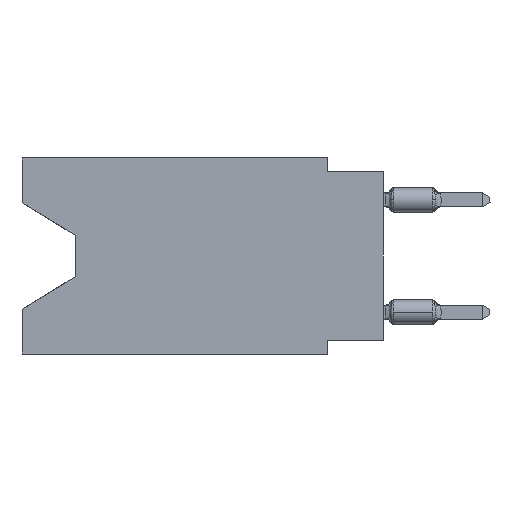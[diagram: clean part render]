
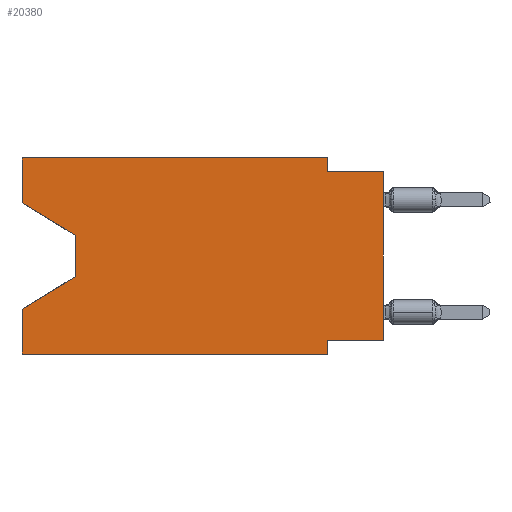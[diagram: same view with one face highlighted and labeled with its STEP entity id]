
A CAD part, left-side view. The second image highlights one B-rep face of the part: STEP entity #20380.
In plain terms, the highlighted planar face has unit normal (-1, 0, 0).
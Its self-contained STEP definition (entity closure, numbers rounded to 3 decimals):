
#86 = CARTESIAN_POINT ( 'NONE',  ( 0., 13.97, -3.505 ) ) ;
#268 = EDGE_CURVE ( 'NONE', #17791, #15368, #21144, .T. ) ;
#581 = CARTESIAN_POINT ( 'NONE',  ( 0., 2.54, 0. ) ) ;
#879 = LINE ( 'NONE', #1012, #8076 ) ;
#906 = CARTESIAN_POINT ( 'NONE',  ( 0., 16.383, -8.89 ) ) ;
#975 = VECTOR ( 'NONE', #2533, 1000. ) ;
#1012 = CARTESIAN_POINT ( 'NONE',  ( 0., 13.97, -3.505 ) ) ;
#1935 = CARTESIAN_POINT ( 'NONE',  ( 0., 16.383, -2.038 ) ) ;
#2030 = ORIENTED_EDGE ( 'NONE', *, *, #5753, .T. ) ;
#2533 = DIRECTION ( 'NONE',  ( 0., 0., 1. ) ) ;
#2632 = CARTESIAN_POINT ( 'NONE',  ( 0., 13.97, -5.385 ) ) ;
#2776 = EDGE_CURVE ( 'NONE', #6403, #15677, #16191, .T. ) ;
#2819 = VECTOR ( 'NONE', #8734, 1000. ) ;
#2836 = ORIENTED_EDGE ( 'NONE', *, *, #17042, .F. ) ;
#2939 = LINE ( 'NONE', #22470, #4425 ) ;
#3413 = DIRECTION ( 'NONE',  ( 0., 1., 0. ) ) ;
#3509 = ORIENTED_EDGE ( 'NONE', *, *, #19777, .T. ) ;
#3523 = ORIENTED_EDGE ( 'NONE', *, *, #9994, .T. ) ;
#3808 = LINE ( 'NONE', #21880, #22168 ) ;
#3850 = VERTEX_POINT ( 'NONE', #581 ) ;
#4386 = EDGE_CURVE ( 'NONE', #15677, #3850, #2939, .T. ) ;
#4425 = VECTOR ( 'NONE', #5489, 1000. ) ;
#4614 = VERTEX_POINT ( 'NONE', #86 ) ;
#5489 = DIRECTION ( 'NONE',  ( 0., -1., 0. ) ) ;
#5656 = CARTESIAN_POINT ( 'NONE',  ( 0., 16.383, 0. ) ) ;
#5742 = EDGE_LOOP ( 'NONE', ( #7027, #24378, #3509, #10641, #2030, #2836, #25265, #3523, #14120, #18488, #19448, #18389 ) ) ;
#5753 = EDGE_CURVE ( 'NONE', #17791, #22949, #25659, .T. ) ;
#5797 = VERTEX_POINT ( 'NONE', #25449 ) ;
#6050 = DIRECTION ( 'NONE',  ( 0., 0., 1. ) ) ;
#6226 = VERTEX_POINT ( 'NONE', #6726 ) ;
#6403 = VERTEX_POINT ( 'NONE', #7394 ) ;
#6479 = DIRECTION ( 'NONE',  ( 0., 0., -1. ) ) ;
#6726 = CARTESIAN_POINT ( 'NONE',  ( 0., 0., -0.635 ) ) ;
#7027 = ORIENTED_EDGE ( 'NONE', *, *, #17648, .T. ) ;
#7394 = CARTESIAN_POINT ( 'NONE',  ( 0., 16.383, -2.038 ) ) ;
#7539 = CARTESIAN_POINT ( 'NONE',  ( 0., 13.97, -5.385 ) ) ;
#8076 = VECTOR ( 'NONE', #21118, 1000. ) ;
#8260 = EDGE_CURVE ( 'NONE', #15096, #6226, #25615, .T. ) ;
#8734 = DIRECTION ( 'NONE',  ( 0., -1., 0. ) ) ;
#9376 = VECTOR ( 'NONE', #10988, 1000. ) ;
#9994 = EDGE_CURVE ( 'NONE', #26076, #6226, #24973, .T. ) ;
#10641 = ORIENTED_EDGE ( 'NONE', *, *, #268, .F. ) ;
#10988 = DIRECTION ( 'NONE',  ( 0., -1., 0. ) ) ;
#11027 = CARTESIAN_POINT ( 'NONE',  ( 0., 16.383, 0. ) ) ;
#11152 = VECTOR ( 'NONE', #15782, 1000. ) ;
#11341 = VERTEX_POINT ( 'NONE', #2632 ) ;
#11679 = CARTESIAN_POINT ( 'NONE',  ( 0., 2.54, -8.89 ) ) ;
#12353 = CARTESIAN_POINT ( 'NONE',  ( 0., 0., 0. ) ) ;
#12594 = CARTESIAN_POINT ( 'NONE',  ( 0., 16.383, -6.852 ) ) ;
#13300 = CARTESIAN_POINT ( 'NONE',  ( 0., 0., -8.255 ) ) ;
#13418 = CARTESIAN_POINT ( 'NONE',  ( 0., 2.54, -0.635 ) ) ;
#14026 = EDGE_CURVE ( 'NONE', #26076, #5797, #3808, .T. ) ;
#14120 = ORIENTED_EDGE ( 'NONE', *, *, #8260, .F. ) ;
#15096 = VERTEX_POINT ( 'NONE', #13418 ) ;
#15368 = VERTEX_POINT ( 'NONE', #12594 ) ;
#15556 = FACE_OUTER_BOUND ( 'NONE', #5742, .T. ) ;
#15677 = VERTEX_POINT ( 'NONE', #24255 ) ;
#15782 = DIRECTION ( 'NONE',  ( 0., 0.855, -0.519 ) ) ;
#15919 = CARTESIAN_POINT ( 'NONE',  ( 0., 2.54, 0. ) ) ;
#16191 = LINE ( 'NONE', #5656, #25421 ) ;
#16354 = VECTOR ( 'NONE', #22291, 1000. ) ;
#16793 = DIRECTION ( 'NONE',  ( 0., 0., 1. ) ) ;
#17042 = EDGE_CURVE ( 'NONE', #5797, #22949, #22516, .T. ) ;
#17623 = VECTOR ( 'NONE', #22230, 1000. ) ;
#17648 = EDGE_CURVE ( 'NONE', #6403, #4614, #24559, .T. ) ;
#17791 = VERTEX_POINT ( 'NONE', #26143 ) ;
#18389 = ORIENTED_EDGE ( 'NONE', *, *, #2776, .F. ) ;
#18424 = VECTOR ( 'NONE', #6479, 1000. ) ;
#18488 = ORIENTED_EDGE ( 'NONE', *, *, #19805, .F. ) ;
#19448 = ORIENTED_EDGE ( 'NONE', *, *, #4386, .F. ) ;
#19777 = EDGE_CURVE ( 'NONE', #11341, #15368, #25957, .T. ) ;
#19805 = EDGE_CURVE ( 'NONE', #3850, #15096, #23969, .T. ) ;
#19868 = DIRECTION ( 'NONE',  ( 1., 0., 0. ) ) ;
#20380 = ADVANCED_FACE ( 'NONE', ( #15556 ), #25991, .F. ) ;
#20774 = CARTESIAN_POINT ( 'NONE',  ( 0., 2.54, -8.89 ) ) ;
#21118 = DIRECTION ( 'NONE',  ( 0., 0., -1. ) ) ;
#21144 = LINE ( 'NONE', #11027, #975 ) ;
#21880 = CARTESIAN_POINT ( 'NONE',  ( 0., 0., -8.255 ) ) ;
#21913 = AXIS2_PLACEMENT_3D ( 'NONE', #23607, #19868, #25471 ) ;
#22168 = VECTOR ( 'NONE', #3413, 1000. ) ;
#22230 = DIRECTION ( 'NONE',  ( 0., 0., -1. ) ) ;
#22291 = DIRECTION ( 'NONE',  ( 0., -0.855, -0.519 ) ) ;
#22346 = VECTOR ( 'NONE', #16793, 1000. ) ;
#22470 = CARTESIAN_POINT ( 'NONE',  ( 0., 16.383, 0. ) ) ;
#22516 = LINE ( 'NONE', #20774, #18424 ) ;
#22949 = VERTEX_POINT ( 'NONE', #11679 ) ;
#23607 = CARTESIAN_POINT ( 'NONE',  ( 0., 16.383, 0. ) ) ;
#23969 = LINE ( 'NONE', #15919, #17623 ) ;
#24255 = CARTESIAN_POINT ( 'NONE',  ( 0., 16.383, 0. ) ) ;
#24378 = ORIENTED_EDGE ( 'NONE', *, *, #26078, .T. ) ;
#24559 = LINE ( 'NONE', #1935, #16354 ) ;
#24973 = LINE ( 'NONE', #12353, #22346 ) ;
#25265 = ORIENTED_EDGE ( 'NONE', *, *, #14026, .F. ) ;
#25421 = VECTOR ( 'NONE', #6050, 1000. ) ;
#25449 = CARTESIAN_POINT ( 'NONE',  ( 0., 2.54, -8.255 ) ) ;
#25471 = DIRECTION ( 'NONE',  ( 0., 0., -1. ) ) ;
#25485 = CARTESIAN_POINT ( 'NONE',  ( 0., 0., -0.635 ) ) ;
#25615 = LINE ( 'NONE', #25485, #9376 ) ;
#25659 = LINE ( 'NONE', #906, #2819 ) ;
#25957 = LINE ( 'NONE', #7539, #11152 ) ;
#25991 = PLANE ( 'NONE',  #21913 ) ;
#26076 = VERTEX_POINT ( 'NONE', #13300 ) ;
#26078 = EDGE_CURVE ( 'NONE', #4614, #11341, #879, .T. ) ;
#26143 = CARTESIAN_POINT ( 'NONE',  ( 0., 16.383, -8.89 ) ) ;
